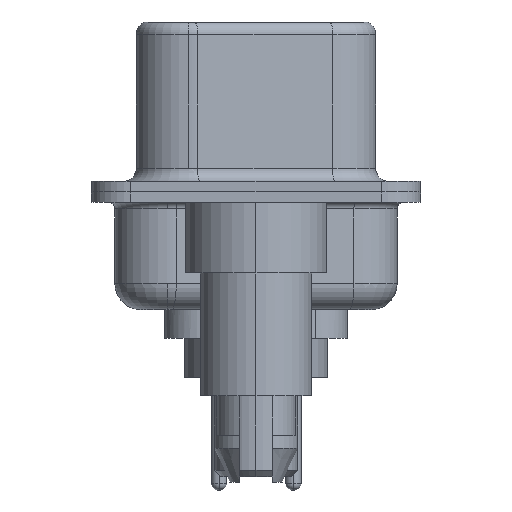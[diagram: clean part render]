
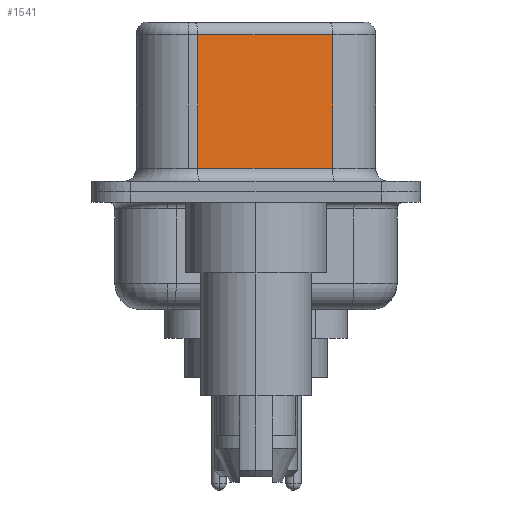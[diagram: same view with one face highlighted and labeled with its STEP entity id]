
A CAD part, left-side view. The second image highlights one B-rep face of the part: STEP entity #1541.
In plain terms, the highlighted planar face has unit normal (-0.985, -0.174, 0).
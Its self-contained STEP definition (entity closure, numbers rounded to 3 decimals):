
#631 = CARTESIAN_POINT ( 'NONE',  ( 4.585, -2.927, 6.02 ) ) ;
#848 = EDGE_CURVE ( 'NONE', #15144, #7536, #17968, .T. ) ;
#1123 = ORIENTED_EDGE ( 'NONE', *, *, #848, .T. ) ;
#1430 = VECTOR ( 'NONE', #13925, 1000. ) ;
#1541 = ADVANCED_FACE ( 'NONE', ( #4902 ), #12487, .F. ) ;
#1890 = VECTOR ( 'NONE', #6231, 1000. ) ;
#2418 = CARTESIAN_POINT ( 'NONE',  ( 4.585, -2.927, 0.9 ) ) ;
#2838 = CARTESIAN_POINT ( 'NONE',  ( 4.585, -2.927, 6.02 ) ) ;
#3228 = DIRECTION ( 'NONE',  ( 0., 0., -1. ) ) ;
#4126 = DIRECTION ( 'NONE',  ( 0.985, 0.174, 0. ) ) ;
#4902 = FACE_OUTER_BOUND ( 'NONE', #9403, .T. ) ;
#5488 = CARTESIAN_POINT ( 'NONE',  ( 4.585, -2.927, 6.52 ) ) ;
#5583 = LINE ( 'NONE', #14619, #1890 ) ;
#5893 = VERTEX_POINT ( 'NONE', #631 ) ;
#6231 = DIRECTION ( 'NONE',  ( 0., 0., -1. ) ) ;
#6445 = VECTOR ( 'NONE', #3228, 1000. ) ;
#6549 = CARTESIAN_POINT ( 'NONE',  ( 3.675, 2.233, 0.9 ) ) ;
#6558 = DIRECTION ( 'NONE',  ( 0.174, -0.985, 0. ) ) ;
#6650 = EDGE_CURVE ( 'NONE', #5893, #7536, #5583, .T. ) ;
#7087 = VERTEX_POINT ( 'NONE', #11784 ) ;
#7536 = VERTEX_POINT ( 'NONE', #8457 ) ;
#7721 = VECTOR ( 'NONE', #6558, 1000. ) ;
#8188 = ORIENTED_EDGE ( 'NONE', *, *, #12321, .T. ) ;
#8457 = CARTESIAN_POINT ( 'NONE',  ( 4.585, -2.927, 0.9 ) ) ;
#9403 = EDGE_LOOP ( 'NONE', ( #17659, #8188, #10842, #1123 ) ) ;
#9708 = LINE ( 'NONE', #11568, #6445 ) ;
#9983 = DIRECTION ( 'NONE',  ( -0.174, 0.985, 0. ) ) ;
#10842 = ORIENTED_EDGE ( 'NONE', *, *, #16629, .T. ) ;
#11568 = CARTESIAN_POINT ( 'NONE',  ( 3.675, 2.233, 6.52 ) ) ;
#11784 = CARTESIAN_POINT ( 'NONE',  ( 3.675, 2.233, 6.02 ) ) ;
#12321 = EDGE_CURVE ( 'NONE', #5893, #7087, #16285, .T. ) ;
#12487 = PLANE ( 'NONE',  #16573 ) ;
#13925 = DIRECTION ( 'NONE',  ( -0.174, 0.985, 0. ) ) ;
#14619 = CARTESIAN_POINT ( 'NONE',  ( 4.585, -2.927, 6.52 ) ) ;
#15144 = VERTEX_POINT ( 'NONE', #6549 ) ;
#16285 = LINE ( 'NONE', #2838, #1430 ) ;
#16573 = AXIS2_PLACEMENT_3D ( 'NONE', #5488, #4126, #9983 ) ;
#16629 = EDGE_CURVE ( 'NONE', #7087, #15144, #9708, .T. ) ;
#17659 = ORIENTED_EDGE ( 'NONE', *, *, #6650, .F. ) ;
#17968 = LINE ( 'NONE', #2418, #7721 ) ;
